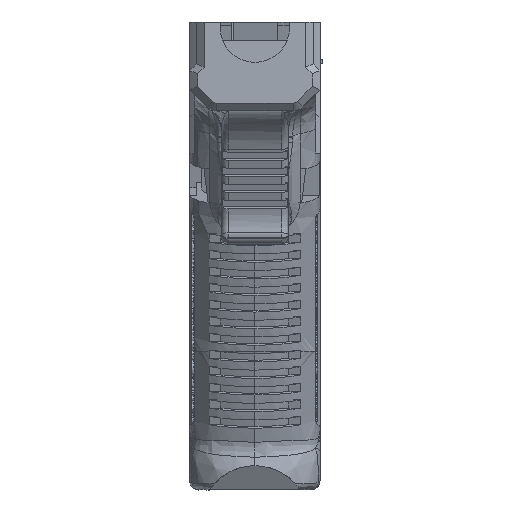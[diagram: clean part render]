
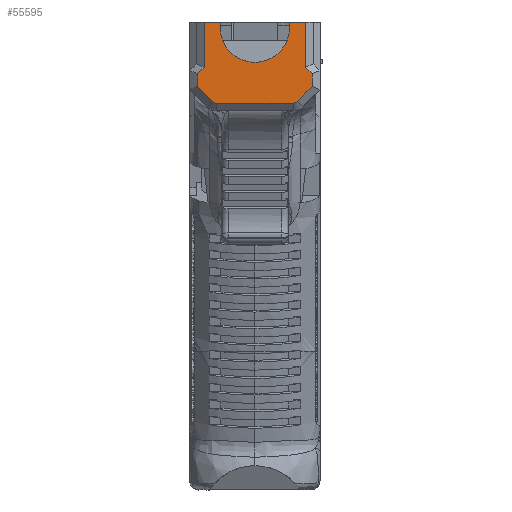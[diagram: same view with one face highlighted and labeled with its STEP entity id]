
A CAD part, left-side view. The second image highlights one B-rep face of the part: STEP entity #55595.
In plain terms, the highlighted planar face has unit normal (-1, 0, 0).
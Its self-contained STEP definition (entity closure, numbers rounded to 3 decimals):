
#6545=PLANE('',#59015);
#7541=B_SPLINE_CURVE_WITH_KNOTS('',3,(#69676,#69677,#69678,#69679),
 .UNSPECIFIED.,.F.,.F.,(4,4),(-0.393,0.393),
 .UNSPECIFIED.);
#7542=B_SPLINE_CURVE_WITH_KNOTS('',3,(#69683,#69684,#69685,#69686),
 .UNSPECIFIED.,.F.,.F.,(4,4),(-0.393,0.393),
 .UNSPECIFIED.);
#8813=FACE_OUTER_BOUND('',#12190,.T.);
#12190=EDGE_LOOP('',(#38475,#38476,#38477,#38478,#38479,#38480,#38481,#38482,
#38483,#38484,#38485,#38486,#38487,#38488,#38489,#38490));
#15928=CIRCLE('',#59016,7.765);
#16208=LINE('',#66741,#19763);
#16219=LINE('',#66765,#19774);
#16409=LINE('',#69655,#19964);
#16413=LINE('',#69662,#19968);
#16414=LINE('',#69666,#19969);
#16415=LINE('',#69668,#19970);
#16416=LINE('',#69670,#19971);
#16417=LINE('',#69672,#19972);
#16418=LINE('',#69674,#19973);
#16419=LINE('',#69681,#19974);
#16420=LINE('',#69688,#19975);
#16421=LINE('',#69690,#19976);
#16422=LINE('',#69691,#19977);
#19763=VECTOR('',#60447,10.);
#19774=VECTOR('',#60464,10.);
#19964=VECTOR('',#60778,10.);
#19968=VECTOR('',#60784,10.);
#19969=VECTOR('',#60789,10.);
#19970=VECTOR('',#60790,10.);
#19971=VECTOR('',#60791,10.);
#19972=VECTOR('',#60792,10.);
#19973=VECTOR('',#60793,10.);
#19974=VECTOR('',#60794,10.);
#19975=VECTOR('',#60795,10.);
#19976=VECTOR('',#60796,10.);
#19977=VECTOR('',#60797,10.);
#23354=VERTEX_POINT('',#66738);
#23355=VERTEX_POINT('',#66740);
#23364=VERTEX_POINT('',#66762);
#23365=VERTEX_POINT('',#66764);
#23594=VERTEX_POINT('',#69654);
#23596=VERTEX_POINT('',#69660);
#23597=VERTEX_POINT('',#69664);
#23598=VERTEX_POINT('',#69667);
#23599=VERTEX_POINT('',#69669);
#23600=VERTEX_POINT('',#69671);
#23601=VERTEX_POINT('',#69673);
#23602=VERTEX_POINT('',#69675);
#23603=VERTEX_POINT('',#69680);
#23604=VERTEX_POINT('',#69682);
#23605=VERTEX_POINT('',#69687);
#23606=VERTEX_POINT('',#69689);
#29207=EDGE_CURVE('',#23354,#23355,#16208,.T.);
#29219=EDGE_CURVE('',#23365,#23364,#16219,.T.);
#29502=EDGE_CURVE('',#23594,#23365,#16409,.T.);
#29506=EDGE_CURVE('',#23596,#23364,#16413,.T.);
#29507=EDGE_CURVE('',#23596,#23597,#15928,.T.);
#29508=EDGE_CURVE('',#23597,#23355,#16414,.T.);
#29509=EDGE_CURVE('',#23598,#23354,#16415,.T.);
#29510=EDGE_CURVE('',#23599,#23598,#16416,.T.);
#29511=EDGE_CURVE('',#23600,#23599,#16417,.T.);
#29512=EDGE_CURVE('',#23601,#23600,#16418,.T.);
#29513=EDGE_CURVE('',#23602,#23601,#7541,.T.);
#29514=EDGE_CURVE('',#23603,#23602,#16419,.T.);
#29515=EDGE_CURVE('',#23604,#23603,#7542,.T.);
#29516=EDGE_CURVE('',#23605,#23604,#16420,.T.);
#29517=EDGE_CURVE('',#23606,#23605,#16421,.T.);
#29518=EDGE_CURVE('',#23594,#23606,#16422,.T.);
#38475=ORIENTED_EDGE('',*,*,#29219,.T.);
#38476=ORIENTED_EDGE('',*,*,#29506,.F.);
#38477=ORIENTED_EDGE('',*,*,#29507,.T.);
#38478=ORIENTED_EDGE('',*,*,#29508,.T.);
#38479=ORIENTED_EDGE('',*,*,#29207,.F.);
#38480=ORIENTED_EDGE('',*,*,#29509,.F.);
#38481=ORIENTED_EDGE('',*,*,#29510,.F.);
#38482=ORIENTED_EDGE('',*,*,#29511,.F.);
#38483=ORIENTED_EDGE('',*,*,#29512,.F.);
#38484=ORIENTED_EDGE('',*,*,#29513,.F.);
#38485=ORIENTED_EDGE('',*,*,#29514,.F.);
#38486=ORIENTED_EDGE('',*,*,#29515,.F.);
#38487=ORIENTED_EDGE('',*,*,#29516,.F.);
#38488=ORIENTED_EDGE('',*,*,#29517,.F.);
#38489=ORIENTED_EDGE('',*,*,#29518,.F.);
#38490=ORIENTED_EDGE('',*,*,#29502,.T.);
#55595=ADVANCED_FACE('',(#8813),#6545,.F.);
#59015=AXIS2_PLACEMENT_3D('',#69663,#60785,#60786);
#59016=AXIS2_PLACEMENT_3D('',#69665,#60787,#60788);
#60447=DIRECTION('',(0.,-1.,0.));
#60464=DIRECTION('',(0.,1.,0.));
#60778=DIRECTION('',(0.,0.,1.));
#60784=DIRECTION('',(0.,0.,1.));
#60785=DIRECTION('center_axis',(1.,0.,
0.));
#60786=DIRECTION('ref_axis',(0.,1.,0.));
#60787=DIRECTION('center_axis',(1.,0.,
0.));
#60788=DIRECTION('ref_axis',(0.,0.,
-1.));
#60789=DIRECTION('',(0.,0.,1.));
#60790=DIRECTION('',(0.,0.,1.));
#60791=DIRECTION('',(0.,-0.707,0.707));
#60792=DIRECTION('',(0.,0.,1.));
#60793=DIRECTION('',(0.,0.707,0.707));
#60794=DIRECTION('',(0.,1.,0.));
#60795=DIRECTION('',(0.,0.707,-0.707));
#60796=DIRECTION('',(0.,0.,-1.));
#60797=DIRECTION('',(0.,-0.707,-0.707));
#66738=CARTESIAN_POINT('',(128.368,-43.784,-24.061));
#66740=CARTESIAN_POINT('',(128.368,-47.386,-24.061));
#66741=CARTESIAN_POINT('',(128.368,-62.763,-24.061));
#66762=CARTESIAN_POINT('',(128.368,-62.914,-24.061));
#66764=CARTESIAN_POINT('',(128.368,-66.516,-24.061));
#66765=CARTESIAN_POINT('',(128.368,-62.763,-24.061));
#69654=CARTESIAN_POINT('',(128.368,-66.516,-34.172));
#69655=CARTESIAN_POINT('',(128.368,-66.516,-23.447));
#69660=CARTESIAN_POINT('',(128.368,-62.914,-25.477));
#69662=CARTESIAN_POINT('',(128.368,-62.914,-23.447));
#69663=CARTESIAN_POINT('Origin',(128.367,-55.151,-76.648));
#69664=CARTESIAN_POINT('',(128.368,-47.386,-25.477));
#69665=CARTESIAN_POINT('Origin',(128.368,-55.15,-25.35));
#69666=CARTESIAN_POINT('',(128.368,-47.386,-50.935));
#69667=CARTESIAN_POINT('',(128.368,-43.784,-34.172));
#69668=CARTESIAN_POINT('',(128.368,-43.784,-50.047));
#69669=CARTESIAN_POINT('',(128.368,-42.284,-35.672));
#69670=CARTESIAN_POINT('',(128.368,-35.376,-42.58));
#69671=CARTESIAN_POINT('',(128.368,-42.284,-38.526));
#69672=CARTESIAN_POINT('',(128.368,-42.284,-50.301));
#69673=CARTESIAN_POINT('',(128.368,-45.643,-41.884));
#69674=CARTESIAN_POINT('',(128.368,-55.962,-52.204));
#69675=CARTESIAN_POINT('',(128.368,-46.527,-42.25));
#69676=CARTESIAN_POINT('Ctrl Pts',(128.368,-46.527,-42.25));
#69677=CARTESIAN_POINT('Ctrl Pts',(128.368,-46.199,-42.25));
#69678=CARTESIAN_POINT('Ctrl Pts',(128.368,-45.874,-42.116));
#69679=CARTESIAN_POINT('Ctrl Pts',(128.368,-45.643,-41.884));
#69680=CARTESIAN_POINT('',(128.368,-63.773,-42.25));
#69681=CARTESIAN_POINT('',(128.368,-55.15,-42.25));
#69682=CARTESIAN_POINT('',(128.368,-64.657,-41.884));
#69683=CARTESIAN_POINT('Ctrl Pts',(128.368,-64.657,-41.884));
#69684=CARTESIAN_POINT('Ctrl Pts',(128.368,-64.426,-42.116));
#69685=CARTESIAN_POINT('Ctrl Pts',(128.368,-64.101,-42.25));
#69686=CARTESIAN_POINT('Ctrl Pts',(128.368,-63.773,-42.25));
#69687=CARTESIAN_POINT('',(128.368,-68.016,-38.526));
#69688=CARTESIAN_POINT('',(128.368,-54.338,-52.203));
#69689=CARTESIAN_POINT('',(128.368,-68.016,-35.672));
#69690=CARTESIAN_POINT('',(128.368,-68.016,-50.301));
#69691=CARTESIAN_POINT('',(128.368,-74.925,-42.581));
